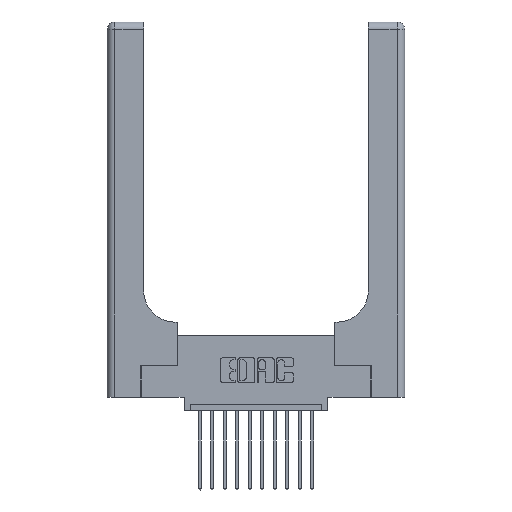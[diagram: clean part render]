
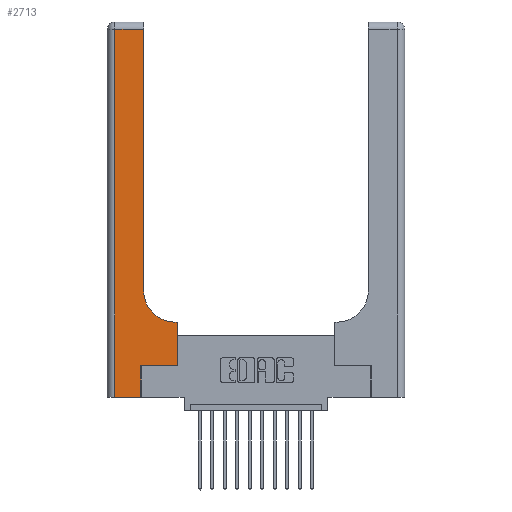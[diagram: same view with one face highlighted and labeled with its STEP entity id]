
A CAD part, top view. The second image highlights one B-rep face of the part: STEP entity #2713.
In plain terms, the highlighted planar face has unit normal (0, 0, 1).
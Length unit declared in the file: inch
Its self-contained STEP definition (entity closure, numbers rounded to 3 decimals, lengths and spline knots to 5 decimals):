
#113 = VECTOR ( 'NONE', #13960, 39.37008 ) ;
#126 = CARTESIAN_POINT ( 'NONE',  ( 0., 0., 0.37 ) ) ;
#264 = EDGE_CURVE ( 'NONE', #12600, #363, #7018, .T. ) ;
#329 = VERTEX_POINT ( 'NONE', #16506 ) ;
#363 = VERTEX_POINT ( 'NONE', #15233 ) ;
#555 = ORIENTED_EDGE ( 'NONE', *, *, #12794, .T. ) ;
#704 = DIRECTION ( 'NONE',  ( 0., 0., -1. ) ) ;
#746 = CARTESIAN_POINT ( 'NONE',  ( 0.269, 0.25, 0.37 ) ) ;
#850 = ORIENTED_EDGE ( 'NONE', *, *, #2063, .T. ) ;
#1526 = DIRECTION ( 'NONE',  ( -1., 0., 0. ) ) ;
#1570 = ORIENTED_EDGE ( 'NONE', *, *, #7097, .T. ) ;
#1613 = DIRECTION ( 'NONE',  ( 0., -1., 0. ) ) ;
#2063 = EDGE_CURVE ( 'NONE', #16035, #5810, #8623, .T. ) ;
#2713 = ADVANCED_FACE ( 'NONE', ( #4069 ), #14072, .F. ) ;
#2841 = VERTEX_POINT ( 'NONE', #6401 ) ;
#3512 = CARTESIAN_POINT ( 'NONE',  ( 0.269, 0.25, 0.37 ) ) ;
#3940 = CARTESIAN_POINT ( 'NONE',  ( 0.5585, 0.25, 0.37 ) ) ;
#4069 = FACE_OUTER_BOUND ( 'NONE', #10154, .T. ) ;
#4388 = LINE ( 'NONE', #3940, #9755 ) ;
#4578 = ORIENTED_EDGE ( 'NONE', *, *, #5864, .T. ) ;
#5365 = VERTEX_POINT ( 'NONE', #13803 ) ;
#5726 = LINE ( 'NONE', #10659, #9044 ) ;
#5810 = VERTEX_POINT ( 'NONE', #6297 ) ;
#5864 = EDGE_CURVE ( 'NONE', #363, #14309, #14941, .T. ) ;
#6065 = CARTESIAN_POINT ( 'NONE',  ( 0.2915, 2.94, 0.37 ) ) ;
#6114 = DIRECTION ( 'NONE',  ( -1., 0., 0. ) ) ;
#6297 = CARTESIAN_POINT ( 'NONE',  ( 0.2915, 0.85, 0.37 ) ) ;
#6337 = AXIS2_PLACEMENT_3D ( 'NONE', #10604, #15862, #11840 ) ;
#6401 = CARTESIAN_POINT ( 'NONE',  ( 0.5585, 0.6, 0.37 ) ) ;
#6506 = CARTESIAN_POINT ( 'NONE',  ( 0.5415, 0.6, 0.37 ) ) ;
#6601 = VECTOR ( 'NONE', #1526, 39.37008 ) ;
#6729 = DIRECTION ( 'NONE',  ( 1., 0., 0. ) ) ;
#7018 = LINE ( 'NONE', #9544, #6601 ) ;
#7097 = EDGE_CURVE ( 'NONE', #329, #13271, #10533, .T. ) ;
#8147 = CARTESIAN_POINT ( 'NONE',  ( 0.06, 3., 0.37 ) ) ;
#8623 = CIRCLE ( 'NONE', #6337, 0.25 ) ;
#9044 = VECTOR ( 'NONE', #10714, 39.37008 ) ;
#9544 = CARTESIAN_POINT ( 'NONE',  ( 0., 2.94, 0.37 ) ) ;
#9755 = VECTOR ( 'NONE', #10448, 39.37008 ) ;
#10127 = LINE ( 'NONE', #126, #14495 ) ;
#10154 = EDGE_LOOP ( 'NONE', ( #12194, #14584, #4578, #11569, #1570, #14412, #555, #15192, #850 ) ) ;
#10373 = EDGE_CURVE ( 'NONE', #2841, #16035, #12939, .T. ) ;
#10392 = VECTOR ( 'NONE', #16727, 39.37008 ) ;
#10448 = DIRECTION ( 'NONE',  ( 0., 1., 0. ) ) ;
#10533 = LINE ( 'NONE', #12461, #14924 ) ;
#10548 = VECTOR ( 'NONE', #1613, 39.37008 ) ;
#10604 = CARTESIAN_POINT ( 'NONE',  ( 0.5415, 0.85, 0.37 ) ) ;
#10659 = CARTESIAN_POINT ( 'NONE',  ( 0.2915, 3., 0.37 ) ) ;
#10714 = DIRECTION ( 'NONE',  ( 0., 1., 0. ) ) ;
#11569 = ORIENTED_EDGE ( 'NONE', *, *, #14923, .T. ) ;
#11840 = DIRECTION ( 'NONE',  ( 1., 0., 0. ) ) ;
#11875 = EDGE_CURVE ( 'NONE', #13271, #5365, #14782, .T. ) ;
#12194 = ORIENTED_EDGE ( 'NONE', *, *, #16756, .T. ) ;
#12461 = CARTESIAN_POINT ( 'NONE',  ( 0.269, 0., 0.37 ) ) ;
#12600 = VERTEX_POINT ( 'NONE', #6065 ) ;
#12794 = EDGE_CURVE ( 'NONE', #5365, #2841, #4388, .T. ) ;
#12939 = LINE ( 'NONE', #13842, #113 ) ;
#13271 = VERTEX_POINT ( 'NONE', #3512 ) ;
#13803 = CARTESIAN_POINT ( 'NONE',  ( 0.5585, 0.25, 0.37 ) ) ;
#13842 = CARTESIAN_POINT ( 'NONE',  ( 0.2915, 0.6, 0.37 ) ) ;
#13930 = DIRECTION ( 'NONE',  ( 0., 1., 0. ) ) ;
#13960 = DIRECTION ( 'NONE',  ( -1., 0., 0. ) ) ;
#14072 = PLANE ( 'NONE',  #15002 ) ;
#14309 = VERTEX_POINT ( 'NONE', #14576 ) ;
#14412 = ORIENTED_EDGE ( 'NONE', *, *, #11875, .T. ) ;
#14495 = VECTOR ( 'NONE', #6729, 39.37008 ) ;
#14576 = CARTESIAN_POINT ( 'NONE',  ( 0.06, 0., 0.37 ) ) ;
#14584 = ORIENTED_EDGE ( 'NONE', *, *, #264, .T. ) ;
#14782 = LINE ( 'NONE', #746, #10392 ) ;
#14923 = EDGE_CURVE ( 'NONE', #14309, #329, #10127, .T. ) ;
#14924 = VECTOR ( 'NONE', #13930, 39.37008 ) ;
#14941 = LINE ( 'NONE', #8147, #10548 ) ;
#15002 = AXIS2_PLACEMENT_3D ( 'NONE', #15235, #704, #6114 ) ;
#15192 = ORIENTED_EDGE ( 'NONE', *, *, #10373, .T. ) ;
#15233 = CARTESIAN_POINT ( 'NONE',  ( 0.06, 2.94, 0.37 ) ) ;
#15235 = CARTESIAN_POINT ( 'NONE',  ( 0., 3., 0.37 ) ) ;
#15862 = DIRECTION ( 'NONE',  ( 0., 0., -1. ) ) ;
#16035 = VERTEX_POINT ( 'NONE', #6506 ) ;
#16506 = CARTESIAN_POINT ( 'NONE',  ( 0.269, 0., 0.37 ) ) ;
#16727 = DIRECTION ( 'NONE',  ( 1., 0., 0. ) ) ;
#16756 = EDGE_CURVE ( 'NONE', #5810, #12600, #5726, .T. ) ;
